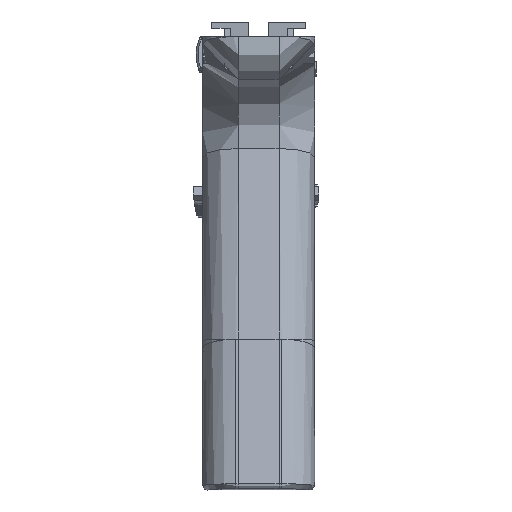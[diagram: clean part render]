
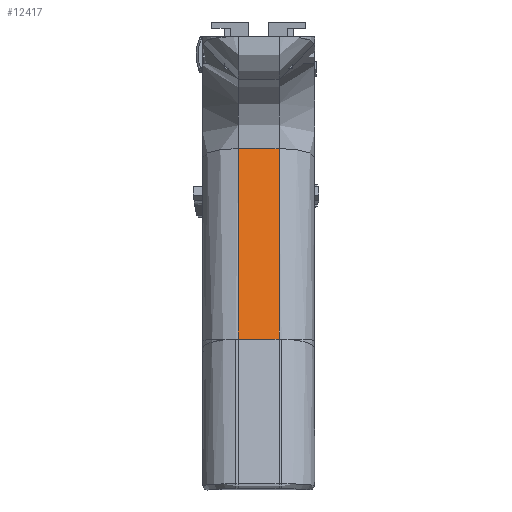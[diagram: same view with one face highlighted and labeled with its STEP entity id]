
A CAD part, front view. The second image highlights one B-rep face of the part: STEP entity #12417.
In plain terms, the highlighted face is planar.
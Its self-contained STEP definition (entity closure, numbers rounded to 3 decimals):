
#901=PLANE('',#13545);
#1480=FACE_OUTER_BOUND('',#2189,.T.);
#2189=EDGE_LOOP('',(#10774,#10775,#10776,#10777));
#3145=LINE('',#21544,#4304);
#3308=LINE('',#22423,#4467);
#3309=LINE('',#22426,#4468);
#3310=LINE('',#22427,#4469);
#4304=VECTOR('',#15991,10.);
#4467=VECTOR('',#16418,10.);
#4468=VECTOR('',#16421,10.);
#4469=VECTOR('',#16422,10.);
#5828=VERTEX_POINT('',#21540);
#5829=VERTEX_POINT('',#21542);
#5980=VERTEX_POINT('',#22401);
#5983=VERTEX_POINT('',#22425);
#7417=EDGE_CURVE('',#5828,#5829,#3145,.T.);
#7657=EDGE_CURVE('',#5828,#5980,#3308,.T.);
#7658=EDGE_CURVE('',#5983,#5829,#3309,.T.);
#7659=EDGE_CURVE('',#5980,#5983,#3310,.T.);
#10774=ORIENTED_EDGE('',*,*,#7658,.F.);
#10775=ORIENTED_EDGE('',*,*,#7659,.F.);
#10776=ORIENTED_EDGE('',*,*,#7657,.F.);
#10777=ORIENTED_EDGE('',*,*,#7417,.T.);
#12417=ADVANCED_FACE('',(#1480),#901,.T.);
#13545=AXIS2_PLACEMENT_3D('',#22424,#16419,#16420);
#15991=DIRECTION('',(0.,-0.249,0.969));
#16418=DIRECTION('',(-1.,0.,0.));
#16419=DIRECTION('center_axis',(0.,-0.969,
-0.249));
#16420=DIRECTION('ref_axis',(0.,-0.249,0.969));
#16421=DIRECTION('',(1.,0.,0.));
#16422=DIRECTION('',(0.,-0.249,0.969));
#21540=CARTESIAN_POINT('',(13.45,-71.634,19.877));
#21542=CARTESIAN_POINT('',(13.45,-83.628,66.536));
#21544=CARTESIAN_POINT('',(13.45,-83.554,66.245));
#22401=CARTESIAN_POINT('',(3.45,-71.634,19.877));
#22423=CARTESIAN_POINT('',(22.175,-71.634,19.877));
#22424=CARTESIAN_POINT('Origin',(22.175,-71.634,19.877));
#22425=CARTESIAN_POINT('',(3.45,-83.628,66.536));
#22426=CARTESIAN_POINT('',(22.175,-83.628,66.536));
#22427=CARTESIAN_POINT('',(3.45,-83.554,66.245));
